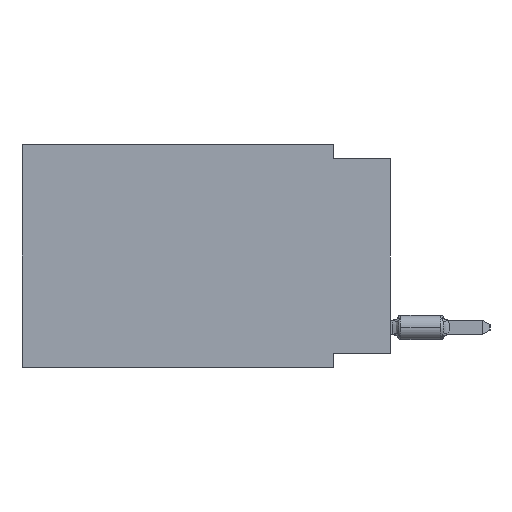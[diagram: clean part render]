
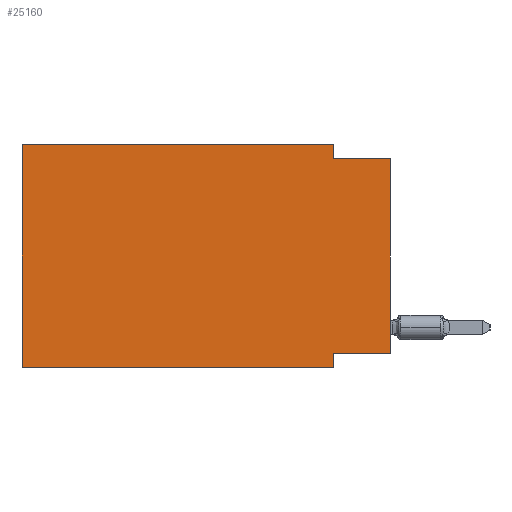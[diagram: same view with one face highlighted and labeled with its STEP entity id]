
A CAD part, left-side view. The second image highlights one B-rep face of the part: STEP entity #25160.
In plain terms, the highlighted planar face has unit normal (-1, 0, 0).
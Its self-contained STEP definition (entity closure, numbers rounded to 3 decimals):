
#187 = CARTESIAN_POINT ( 'NONE',  ( 0., 16.383, 0. ) ) ;
#269 = EDGE_CURVE ( 'NONE', #1002, #4572, #16289, .T. ) ;
#829 = ORIENTED_EDGE ( 'NONE', *, *, #9536, .F. ) ;
#1002 = VERTEX_POINT ( 'NONE', #17947 ) ;
#1868 = EDGE_CURVE ( 'NONE', #20597, #21137, #24833, .T. ) ;
#2132 = VERTEX_POINT ( 'NONE', #18377 ) ;
#2391 = VECTOR ( 'NONE', #13587, 1000. ) ;
#2430 = VERTEX_POINT ( 'NONE', #9508 ) ;
#2605 = CARTESIAN_POINT ( 'NONE',  ( 0., 2.54, 0. ) ) ;
#2757 = LINE ( 'NONE', #17206, #20112 ) ;
#3671 = CARTESIAN_POINT ( 'NONE',  ( 0., 2.54, -9.271 ) ) ;
#3851 = DIRECTION ( 'NONE',  ( 0., -1., 0. ) ) ;
#4301 = DIRECTION ( 'NONE',  ( 1., 0., 0. ) ) ;
#4488 = VECTOR ( 'NONE', #3851, 1000. ) ;
#4572 = VERTEX_POINT ( 'NONE', #2605 ) ;
#5856 = EDGE_CURVE ( 'NONE', #2132, #21137, #21599, .T. ) ;
#6188 = ORIENTED_EDGE ( 'NONE', *, *, #7727, .F. ) ;
#6300 = PLANE ( 'NONE',  #14281 ) ;
#7727 = EDGE_CURVE ( 'NONE', #2132, #1002, #24423, .T. ) ;
#7819 = LINE ( 'NONE', #23762, #2391 ) ;
#8111 = LINE ( 'NONE', #16276, #15411 ) ;
#8638 = DIRECTION ( 'NONE',  ( 0., -1., 0. ) ) ;
#8866 = ORIENTED_EDGE ( 'NONE', *, *, #5856, .T. ) ;
#9283 = EDGE_CURVE ( 'NONE', #23105, #2430, #8111, .T. ) ;
#9508 = CARTESIAN_POINT ( 'NONE',  ( 0., 0., -0.635 ) ) ;
#9536 = EDGE_CURVE ( 'NONE', #24947, #2430, #2757, .T. ) ;
#11221 = CARTESIAN_POINT ( 'NONE',  ( 0., 0., -9.271 ) ) ;
#12396 = DIRECTION ( 'NONE',  ( 0., 0., 1. ) ) ;
#12564 = VECTOR ( 'NONE', #16342, 1000. ) ;
#12581 = FACE_OUTER_BOUND ( 'NONE', #26269, .T. ) ;
#13100 = EDGE_CURVE ( 'NONE', #23105, #20597, #7819, .T. ) ;
#13587 = DIRECTION ( 'NONE',  ( 0., 1., 0. ) ) ;
#14054 = DIRECTION ( 'NONE',  ( 0., -1., 0. ) ) ;
#14281 = AXIS2_PLACEMENT_3D ( 'NONE', #18481, #4301, #24644 ) ;
#15095 = ORIENTED_EDGE ( 'NONE', *, *, #13100, .F. ) ;
#15411 = VECTOR ( 'NONE', #12396, 1000. ) ;
#16015 = VECTOR ( 'NONE', #20680, 1000. ) ;
#16266 = VECTOR ( 'NONE', #18526, 1000. ) ;
#16276 = CARTESIAN_POINT ( 'NONE',  ( 0., 0., 0. ) ) ;
#16289 = LINE ( 'NONE', #24207, #4488 ) ;
#16342 = DIRECTION ( 'NONE',  ( 0., 0., -1. ) ) ;
#17206 = CARTESIAN_POINT ( 'NONE',  ( 0., 0., -0.635 ) ) ;
#17241 = ORIENTED_EDGE ( 'NONE', *, *, #9283, .T. ) ;
#17947 = CARTESIAN_POINT ( 'NONE',  ( 0., 16.383, 0. ) ) ;
#18377 = CARTESIAN_POINT ( 'NONE',  ( 0., 16.383, -9.906 ) ) ;
#18481 = CARTESIAN_POINT ( 'NONE',  ( 0., 16.383, 0. ) ) ;
#18526 = DIRECTION ( 'NONE',  ( 0., 0., 1. ) ) ;
#18624 = CARTESIAN_POINT ( 'NONE',  ( 0., 2.54, 0. ) ) ;
#19060 = CARTESIAN_POINT ( 'NONE',  ( 0., 2.54, -9.906 ) ) ;
#20112 = VECTOR ( 'NONE', #8638, 1000. ) ;
#20225 = LINE ( 'NONE', #18624, #12564 ) ;
#20248 = CARTESIAN_POINT ( 'NONE',  ( 0., 2.54, -9.906 ) ) ;
#20597 = VERTEX_POINT ( 'NONE', #3671 ) ;
#20680 = DIRECTION ( 'NONE',  ( 0., 0., -1. ) ) ;
#20996 = ORIENTED_EDGE ( 'NONE', *, *, #1868, .F. ) ;
#21137 = VERTEX_POINT ( 'NONE', #20248 ) ;
#21466 = CARTESIAN_POINT ( 'NONE',  ( 0., 16.383, -9.906 ) ) ;
#21599 = LINE ( 'NONE', #21466, #25839 ) ;
#22109 = ORIENTED_EDGE ( 'NONE', *, *, #26327, .F. ) ;
#23105 = VERTEX_POINT ( 'NONE', #11221 ) ;
#23762 = CARTESIAN_POINT ( 'NONE',  ( 0., 0., -9.271 ) ) ;
#24207 = CARTESIAN_POINT ( 'NONE',  ( 0., 16.383, 0. ) ) ;
#24423 = LINE ( 'NONE', #187, #16266 ) ;
#24460 = ORIENTED_EDGE ( 'NONE', *, *, #269, .F. ) ;
#24644 = DIRECTION ( 'NONE',  ( 0., 0., -1. ) ) ;
#24833 = LINE ( 'NONE', #19060, #16015 ) ;
#24947 = VERTEX_POINT ( 'NONE', #25199 ) ;
#25160 = ADVANCED_FACE ( 'NONE', ( #12581 ), #6300, .F. ) ;
#25199 = CARTESIAN_POINT ( 'NONE',  ( 0., 2.54, -0.635 ) ) ;
#25839 = VECTOR ( 'NONE', #14054, 1000. ) ;
#26269 = EDGE_LOOP ( 'NONE', ( #17241, #829, #22109, #24460, #6188, #8866, #20996, #15095 ) ) ;
#26327 = EDGE_CURVE ( 'NONE', #4572, #24947, #20225, .T. ) ;
